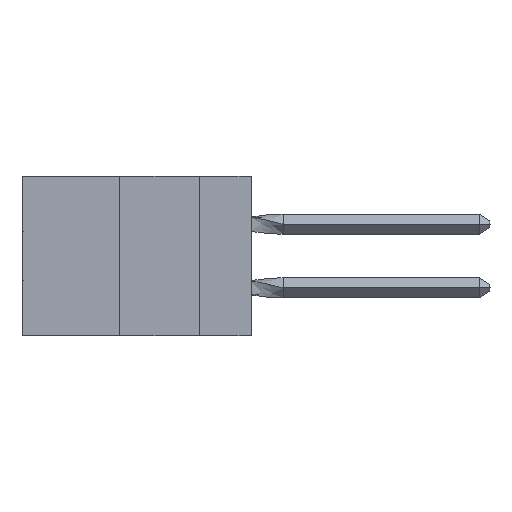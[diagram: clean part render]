
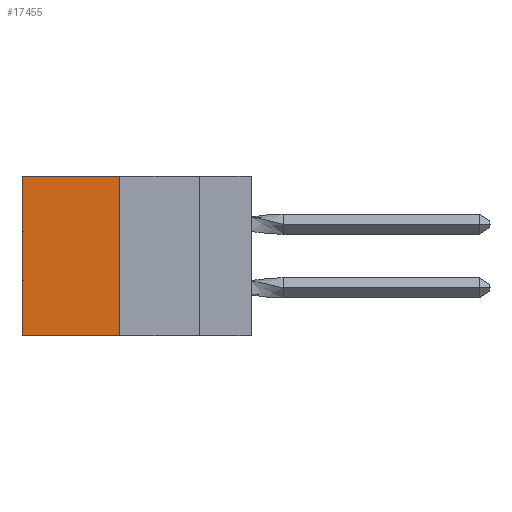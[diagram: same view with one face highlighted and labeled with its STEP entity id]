
A CAD part, left-side view. The second image highlights one B-rep face of the part: STEP entity #17455.
In plain terms, the highlighted planar face has unit normal (-1, 0, 0).
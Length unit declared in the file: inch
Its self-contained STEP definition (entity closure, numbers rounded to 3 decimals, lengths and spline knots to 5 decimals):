
#1972 = CARTESIAN_POINT ( 'NONE',  ( 0.305, 0.72, 0. ) ) ;
#2333 = DIRECTION ( 'NONE',  ( 0., 1., 0. ) ) ;
#5746 = DIRECTION ( 'NONE',  ( 0., 1., 0. ) ) ;
#6263 = DIRECTION ( 'NONE',  ( 1., 0., 0. ) ) ;
#7130 = CARTESIAN_POINT ( 'NONE',  ( 0.305, 0.72, -0.5 ) ) ;
#7707 = FACE_OUTER_BOUND ( 'NONE', #38430, .T. ) ;
#8698 = VECTOR ( 'NONE', #5746, 39.37008 ) ;
#9574 = VECTOR ( 'NONE', #23902, 39.37008 ) ;
#9675 = DIRECTION ( 'NONE',  ( 0., 0., -1. ) ) ;
#9989 = LINE ( 'NONE', #22814, #34404 ) ;
#11375 = AXIS2_PLACEMENT_3D ( 'NONE', #37015, #6263, #9675 ) ;
#12097 = EDGE_CURVE ( 'NONE', #19080, #17398, #9989, .T. ) ;
#14755 = CARTESIAN_POINT ( 'NONE',  ( 0.305, 0.72, -0.5 ) ) ;
#16982 = ORIENTED_EDGE ( 'NONE', *, *, #23417, .F. ) ;
#17263 = CARTESIAN_POINT ( 'NONE',  ( 0.305, 0.413, -0.5 ) ) ;
#17398 = VERTEX_POINT ( 'NONE', #1972 ) ;
#17455 = ADVANCED_FACE ( 'NONE', ( #7707 ), #43393, .F. ) ;
#19080 = VERTEX_POINT ( 'NONE', #30182 ) ;
#20815 = ORIENTED_EDGE ( 'NONE', *, *, #37968, .F. ) ;
#22814 = CARTESIAN_POINT ( 'NONE',  ( 0.305, 0.413, 0. ) ) ;
#23417 = EDGE_CURVE ( 'NONE', #19080, #32100, #41959, .T. ) ;
#23902 = DIRECTION ( 'NONE',  ( 0., 0., -1. ) ) ;
#25083 = LINE ( 'NONE', #39604, #8698 ) ;
#28636 = CARTESIAN_POINT ( 'NONE',  ( 0.305, 0.413, -0.5 ) ) ;
#28997 = EDGE_CURVE ( 'NONE', #17398, #35585, #35578, .T. ) ;
#30182 = CARTESIAN_POINT ( 'NONE',  ( 0.305, 0.413, 0. ) ) ;
#30737 = ORIENTED_EDGE ( 'NONE', *, *, #28997, .T. ) ;
#32100 = VERTEX_POINT ( 'NONE', #28636 ) ;
#32881 = VECTOR ( 'NONE', #34004, 39.37008 ) ;
#34004 = DIRECTION ( 'NONE',  ( 0., 0., -1. ) ) ;
#34404 = VECTOR ( 'NONE', #2333, 39.37008 ) ;
#35578 = LINE ( 'NONE', #7130, #9574 ) ;
#35585 = VERTEX_POINT ( 'NONE', #14755 ) ;
#37015 = CARTESIAN_POINT ( 'NONE',  ( 0.305, 0.413, -0.5 ) ) ;
#37968 = EDGE_CURVE ( 'NONE', #32100, #35585, #25083, .T. ) ;
#38430 = EDGE_LOOP ( 'NONE', ( #30737, #20815, #16982, #38551 ) ) ;
#38551 = ORIENTED_EDGE ( 'NONE', *, *, #12097, .T. ) ;
#39604 = CARTESIAN_POINT ( 'NONE',  ( 0.305, 0.413, -0.5 ) ) ;
#41959 = LINE ( 'NONE', #17263, #32881 ) ;
#43393 = PLANE ( 'NONE',  #11375 ) ;
